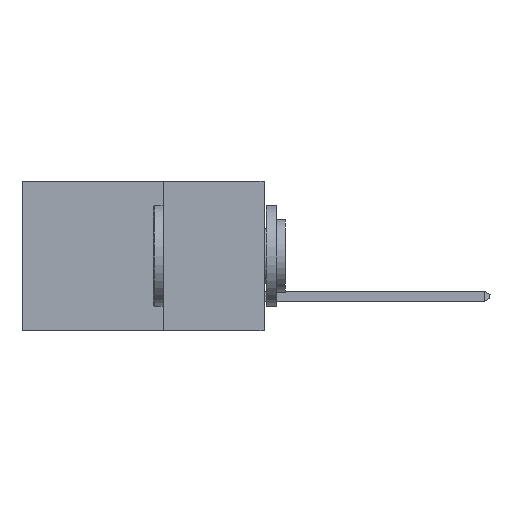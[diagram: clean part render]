
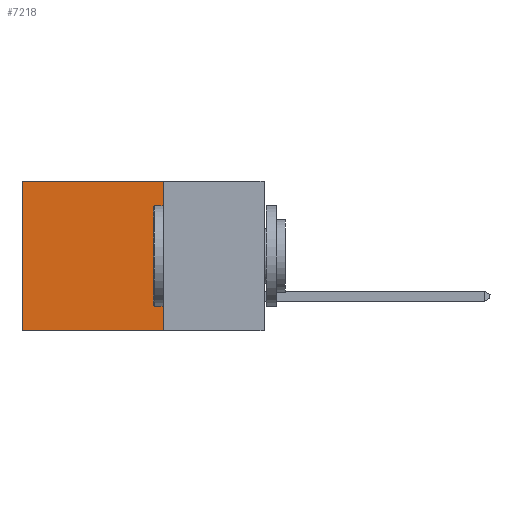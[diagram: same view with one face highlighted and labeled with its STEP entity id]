
A CAD part, left-side view. The second image highlights one B-rep face of the part: STEP entity #7218.
In plain terms, the highlighted planar face has unit normal (-1, 0, 0).
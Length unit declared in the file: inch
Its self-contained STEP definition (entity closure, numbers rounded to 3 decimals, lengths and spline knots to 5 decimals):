
#97 = LINE ( 'NONE', #5105, #1310 ) ;
#276 = LINE ( 'NONE', #11358, #10321 ) ;
#571 = DIRECTION ( 'NONE',  ( 0., 0., -1. ) ) ;
#1310 = VECTOR ( 'NONE', #12743, 39.37008 ) ;
#1884 = EDGE_CURVE ( 'NONE', #2801, #6314, #276, .T. ) ;
#2057 = PLANE ( 'NONE',  #11212 ) ;
#2279 = EDGE_LOOP ( 'NONE', ( #7848, #4718, #13084, #15330 ) ) ;
#2801 = VERTEX_POINT ( 'NONE', #14621 ) ;
#4062 = EDGE_CURVE ( 'NONE', #11914, #6314, #5123, .T. ) ;
#4718 = ORIENTED_EDGE ( 'NONE', *, *, #1884, .F. ) ;
#4754 = EDGE_CURVE ( 'NONE', #8180, #2801, #8306, .T. ) ;
#5105 = CARTESIAN_POINT ( 'NONE',  ( 0.2615, 0.25, 0. ) ) ;
#5123 = LINE ( 'NONE', #12591, #9096 ) ;
#5165 = VECTOR ( 'NONE', #571, 39.37008 ) ;
#6026 = EDGE_CURVE ( 'NONE', #8180, #11914, #97, .T. ) ;
#6314 = VERTEX_POINT ( 'NONE', #14418 ) ;
#7218 = ADVANCED_FACE ( 'NONE', ( #12067 ), #2057, .F. ) ;
#7583 = CARTESIAN_POINT ( 'NONE',  ( 0.2615, 0.25, 0. ) ) ;
#7848 = ORIENTED_EDGE ( 'NONE', *, *, #4062, .T. ) ;
#8180 = VERTEX_POINT ( 'NONE', #7583 ) ;
#8306 = LINE ( 'NONE', #14366, #5165 ) ;
#8381 = DIRECTION ( 'NONE',  ( 0., 0., -1. ) ) ;
#8614 = DIRECTION ( 'NONE',  ( 1., 0., 0. ) ) ;
#8832 = DIRECTION ( 'NONE',  ( 0., 0., -1. ) ) ;
#8906 = CARTESIAN_POINT ( 'NONE',  ( 0.2615, 0.6, 0. ) ) ;
#9096 = VECTOR ( 'NONE', #8832, 39.37008 ) ;
#10321 = VECTOR ( 'NONE', #13898, 39.37008 ) ;
#11212 = AXIS2_PLACEMENT_3D ( 'NONE', #12228, #8614, #8381 ) ;
#11358 = CARTESIAN_POINT ( 'NONE',  ( 0.2615, 0.25, -0.37 ) ) ;
#11914 = VERTEX_POINT ( 'NONE', #8906 ) ;
#12067 = FACE_OUTER_BOUND ( 'NONE', #2279, .T. ) ;
#12228 = CARTESIAN_POINT ( 'NONE',  ( 0.2615, 0.25, -0.37 ) ) ;
#12591 = CARTESIAN_POINT ( 'NONE',  ( 0.2615, 0.6, -0.37 ) ) ;
#12743 = DIRECTION ( 'NONE',  ( 0., 1., 0. ) ) ;
#13084 = ORIENTED_EDGE ( 'NONE', *, *, #4754, .F. ) ;
#13898 = DIRECTION ( 'NONE',  ( 0., 1., 0. ) ) ;
#14366 = CARTESIAN_POINT ( 'NONE',  ( 0.2615, 0.25, -0.37 ) ) ;
#14418 = CARTESIAN_POINT ( 'NONE',  ( 0.2615, 0.6, -0.37 ) ) ;
#14621 = CARTESIAN_POINT ( 'NONE',  ( 0.2615, 0.25, -0.37 ) ) ;
#15330 = ORIENTED_EDGE ( 'NONE', *, *, #6026, .T. ) ;
